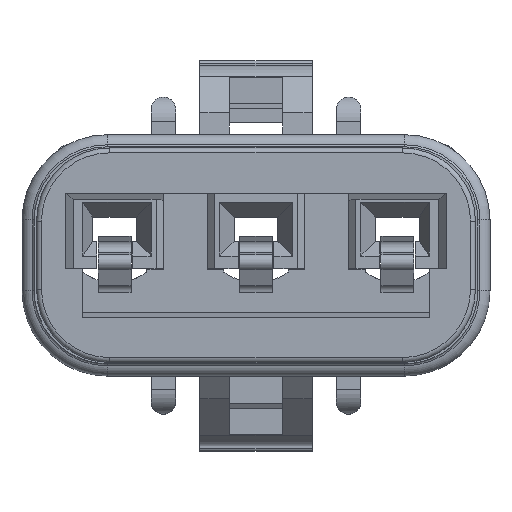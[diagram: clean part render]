
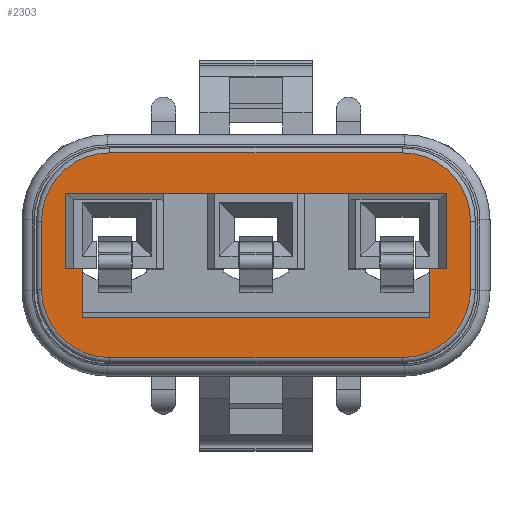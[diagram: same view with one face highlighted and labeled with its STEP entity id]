
A CAD part, top view. The second image highlights one B-rep face of the part: STEP entity #2303.
In plain terms, the highlighted planar face has unit normal (0, 0, 1).
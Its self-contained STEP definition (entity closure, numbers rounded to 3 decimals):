
#38 = LINE ( 'NONE', #7798, #20823 ) ;
#109 = DIRECTION ( 'NONE',  ( 1., 0., 0. ) ) ;
#239 = VERTEX_POINT ( 'NONE', #13555 ) ;
#550 = AXIS2_PLACEMENT_3D ( 'NONE', #7177, #14889, #13173 ) ;
#877 = EDGE_CURVE ( 'NONE', #4485, #15573, #5748, .T. ) ;
#1048 = LINE ( 'NONE', #8560, #22111 ) ;
#1400 = DIRECTION ( 'NONE',  ( 0., 0., 1. ) ) ;
#1514 = VERTEX_POINT ( 'NONE', #10107 ) ;
#1701 = ORIENTED_EDGE ( 'NONE', *, *, #2862, .T. ) ;
#2139 = CIRCLE ( 'NONE', #550, 2.8 ) ;
#2151 = DIRECTION ( 'NONE',  ( 0., 1., 0. ) ) ;
#2303 = ADVANCED_FACE ( 'NONE', ( #15223, #13519 ), #15350, .T. ) ;
#2514 = CARTESIAN_POINT ( 'NONE',  ( 7.125, -0.55, 1.2 ) ) ;
#2654 = DIRECTION ( 'NONE',  ( -1., 0., 0. ) ) ;
#2862 = EDGE_CURVE ( 'NONE', #23455, #21978, #38, .T. ) ;
#3088 = VECTOR ( 'NONE', #14146, 1000. ) ;
#3178 = ORIENTED_EDGE ( 'NONE', *, *, #19509, .T. ) ;
#3377 = CARTESIAN_POINT ( 'NONE',  ( -6., -1.4, 1.2 ) ) ;
#3562 = ORIENTED_EDGE ( 'NONE', *, *, #9195, .T. ) ;
#3669 = EDGE_CURVE ( 'NONE', #9676, #16053, #5112, .T. ) ;
#4128 = DIRECTION ( 'NONE',  ( 1., 0., 0. ) ) ;
#4345 = CARTESIAN_POINT ( 'NONE',  ( -7.825, 2.55, 1.2 ) ) ;
#4485 = VERTEX_POINT ( 'NONE', #19226 ) ;
#4570 = CARTESIAN_POINT ( 'NONE',  ( 3.8, 2.55, 1.2 ) ) ;
#4646 = VERTEX_POINT ( 'NONE', #2514 ) ;
#4940 = DIRECTION ( 'NONE',  ( 1., 0., 0. ) ) ;
#5112 = LINE ( 'NONE', #12576, #19773 ) ;
#5360 = ORIENTED_EDGE ( 'NONE', *, *, #10453, .T. ) ;
#5530 = EDGE_CURVE ( 'NONE', #18386, #4485, #22423, .T. ) ;
#5543 = CIRCLE ( 'NONE', #11796, 2.8 ) ;
#5666 = DIRECTION ( 'NONE',  ( -1., 0., 0. ) ) ;
#5748 = LINE ( 'NONE', #21056, #17946 ) ;
#5795 = DIRECTION ( 'NONE',  ( 0., 0., 1. ) ) ;
#5813 = VECTOR ( 'NONE', #16534, 1000. ) ;
#6271 = EDGE_CURVE ( 'NONE', #23875, #12919, #15872, .T. ) ;
#6560 = DIRECTION ( 'NONE',  ( 0., -1., 0. ) ) ;
#6587 = VERTEX_POINT ( 'NONE', #22367 ) ;
#6703 = VECTOR ( 'NONE', #6560, 1000. ) ;
#7062 = CARTESIAN_POINT ( 'NONE',  ( 6., 1.4, 1.2 ) ) ;
#7071 = CARTESIAN_POINT ( 'NONE',  ( 6., -4.2, 1.2 ) ) ;
#7177 = CARTESIAN_POINT ( 'NONE',  ( 6., -1.4, 1.2 ) ) ;
#7275 = DIRECTION ( 'NONE',  ( 0., -1., 0. ) ) ;
#7515 = VECTOR ( 'NONE', #4128, 1000. ) ;
#7584 = DIRECTION ( 'NONE',  ( 0., 1., 0. ) ) ;
#7798 = CARTESIAN_POINT ( 'NONE',  ( -6., -4.2, 1.2 ) ) ;
#7808 = CARTESIAN_POINT ( 'NONE',  ( 7.125, -2.55, 1.2 ) ) ;
#7863 = VERTEX_POINT ( 'NONE', #8949 ) ;
#8377 = LINE ( 'NONE', #13664, #6703 ) ;
#8509 = CARTESIAN_POINT ( 'NONE',  ( 7.825, 2.55, 1.2 ) ) ;
#8560 = CARTESIAN_POINT ( 'NONE',  ( 7.825, 2.55, 1.2 ) ) ;
#8636 = CARTESIAN_POINT ( 'NONE',  ( -6., -4.2, 1.2 ) ) ;
#8649 = EDGE_CURVE ( 'NONE', #4646, #12919, #12564, .T. ) ;
#8905 = ORIENTED_EDGE ( 'NONE', *, *, #19191, .T. ) ;
#8949 = CARTESIAN_POINT ( 'NONE',  ( 6., 4.2, 1.2 ) ) ;
#8980 = CARTESIAN_POINT ( 'NONE',  ( -7.825, 2.55, 1.2 ) ) ;
#9194 = ORIENTED_EDGE ( 'NONE', *, *, #23990, .T. ) ;
#9195 = EDGE_CURVE ( 'NONE', #7863, #239, #22714, .T. ) ;
#9627 = VERTEX_POINT ( 'NONE', #4570 ) ;
#9676 = VERTEX_POINT ( 'NONE', #8980 ) ;
#9981 = DIRECTION ( 'NONE',  ( 0., -1., 0. ) ) ;
#10107 = CARTESIAN_POINT ( 'NONE',  ( 8.8, 1.4, 1.2 ) ) ;
#10325 = AXIS2_PLACEMENT_3D ( 'NONE', #11915, #5795, #109 ) ;
#10453 = EDGE_CURVE ( 'NONE', #14845, #23455, #21172, .T. ) ;
#10591 = AXIS2_PLACEMENT_3D ( 'NONE', #3377, #1400, #16771 ) ;
#10908 = CARTESIAN_POINT ( 'NONE',  ( -7.825, -0.55, 1.2 ) ) ;
#11796 = AXIS2_PLACEMENT_3D ( 'NONE', #7062, #14649, #14529 ) ;
#11915 = CARTESIAN_POINT ( 'NONE',  ( 0., 0., 1.2 ) ) ;
#12341 = DIRECTION ( 'NONE',  ( 1., 0., 0. ) ) ;
#12399 = ORIENTED_EDGE ( 'NONE', *, *, #8649, .F. ) ;
#12533 = LINE ( 'NONE', #16461, #21524 ) ;
#12564 = LINE ( 'NONE', #23982, #19431 ) ;
#12576 = CARTESIAN_POINT ( 'NONE',  ( -7.825, 2.55, 1.2 ) ) ;
#12788 = CARTESIAN_POINT ( 'NONE',  ( -8.8, 1.4, 1.2 ) ) ;
#12919 = VERTEX_POINT ( 'NONE', #14762 ) ;
#13107 = DIRECTION ( 'NONE',  ( 0., 0., 1. ) ) ;
#13173 = DIRECTION ( 'NONE',  ( 0., -1., 0. ) ) ;
#13327 = DIRECTION ( 'NONE',  ( -1., 0., 0. ) ) ;
#13329 = ORIENTED_EDGE ( 'NONE', *, *, #5530, .T. ) ;
#13334 = ORIENTED_EDGE ( 'NONE', *, *, #877, .T. ) ;
#13519 = FACE_OUTER_BOUND ( 'NONE', #17532, .T. ) ;
#13555 = CARTESIAN_POINT ( 'NONE',  ( -6., 4.2, 1.2 ) ) ;
#13556 = LINE ( 'NONE', #4345, #15757 ) ;
#13664 = CARTESIAN_POINT ( 'NONE',  ( 7.125, -0.55, 1.2 ) ) ;
#13827 = CARTESIAN_POINT ( 'NONE',  ( -7.825, -0.55, 1.2 ) ) ;
#13944 = ORIENTED_EDGE ( 'NONE', *, *, #17935, .T. ) ;
#14146 = DIRECTION ( 'NONE',  ( 0., -1., 0. ) ) ;
#14278 = VECTOR ( 'NONE', #7275, 1000. ) ;
#14529 = DIRECTION ( 'NONE',  ( 1., 0., 0. ) ) ;
#14649 = DIRECTION ( 'NONE',  ( 0., 0., 1. ) ) ;
#14762 = CARTESIAN_POINT ( 'NONE',  ( 7.825, -0.55, 1.2 ) ) ;
#14845 = VERTEX_POINT ( 'NONE', #19666 ) ;
#14889 = DIRECTION ( 'NONE',  ( 0., 0., 1. ) ) ;
#14981 = ORIENTED_EDGE ( 'NONE', *, *, #16760, .T. ) ;
#15223 = FACE_BOUND ( 'NONE', #17785, .T. ) ;
#15350 = PLANE ( 'NONE',  #10325 ) ;
#15539 = ORIENTED_EDGE ( 'NONE', *, *, #20038, .F. ) ;
#15573 = VERTEX_POINT ( 'NONE', #17230 ) ;
#15757 = VECTOR ( 'NONE', #9981, 1000. ) ;
#15872 = LINE ( 'NONE', #8509, #3088 ) ;
#16053 = VERTEX_POINT ( 'NONE', #18349 ) ;
#16461 = CARTESIAN_POINT ( 'NONE',  ( -3.8, 2.55, 1.2 ) ) ;
#16534 = DIRECTION ( 'NONE',  ( 0., 1., 0. ) ) ;
#16760 = EDGE_CURVE ( 'NONE', #22940, #1514, #18366, .T. ) ;
#16771 = DIRECTION ( 'NONE',  ( -1., 0., 0. ) ) ;
#17230 = CARTESIAN_POINT ( 'NONE',  ( -7.125, -0.55, 1.2 ) ) ;
#17297 = CIRCLE ( 'NONE', #19259, 2.8 ) ;
#17355 = VERTEX_POINT ( 'NONE', #10908 ) ;
#17377 = LINE ( 'NONE', #13827, #7515 ) ;
#17532 = EDGE_LOOP ( 'NONE', ( #8905, #3562, #3178, #9194, #5360, #1701, #21529, #14981 ) ) ;
#17785 = EDGE_LOOP ( 'NONE', ( #13334, #18078, #15539, #18946, #13944, #22602, #24134, #12399, #18398, #13329 ) ) ;
#17935 = EDGE_CURVE ( 'NONE', #16053, #9627, #12533, .T. ) ;
#17946 = VECTOR ( 'NONE', #7584, 1000. ) ;
#18078 = ORIENTED_EDGE ( 'NONE', *, *, #19645, .F. ) ;
#18349 = CARTESIAN_POINT ( 'NONE',  ( -3.8, 2.55, 1.2 ) ) ;
#18366 = LINE ( 'NONE', #20446, #5813 ) ;
#18386 = VERTEX_POINT ( 'NONE', #19620 ) ;
#18398 = ORIENTED_EDGE ( 'NONE', *, *, #18498, .T. ) ;
#18451 = DIRECTION ( 'NONE',  ( 1., 0., 0. ) ) ;
#18498 = EDGE_CURVE ( 'NONE', #4646, #18386, #8377, .T. ) ;
#18946 = ORIENTED_EDGE ( 'NONE', *, *, #3669, .T. ) ;
#18981 = CARTESIAN_POINT ( 'NONE',  ( -6., 1.4, 1.2 ) ) ;
#19030 = CARTESIAN_POINT ( 'NONE',  ( 6., 4.2, 1.2 ) ) ;
#19146 = VECTOR ( 'NONE', #13327, 1000. ) ;
#19191 = EDGE_CURVE ( 'NONE', #1514, #7863, #5543, .T. ) ;
#19226 = CARTESIAN_POINT ( 'NONE',  ( -7.125, -2.55, 1.2 ) ) ;
#19259 = AXIS2_PLACEMENT_3D ( 'NONE', #18981, #13107, #2151 ) ;
#19431 = VECTOR ( 'NONE', #18451, 1000. ) ;
#19509 = EDGE_CURVE ( 'NONE', #239, #6587, #17297, .T. ) ;
#19512 = CARTESIAN_POINT ( 'NONE',  ( 8.8, -1.4, 1.2 ) ) ;
#19620 = CARTESIAN_POINT ( 'NONE',  ( 7.125, -2.55, 1.2 ) ) ;
#19645 = EDGE_CURVE ( 'NONE', #17355, #15573, #17377, .T. ) ;
#19666 = CARTESIAN_POINT ( 'NONE',  ( -8.8, -1.4, 1.2 ) ) ;
#19773 = VECTOR ( 'NONE', #12341, 1000. ) ;
#20038 = EDGE_CURVE ( 'NONE', #9676, #17355, #13556, .T. ) ;
#20446 = CARTESIAN_POINT ( 'NONE',  ( 8.8, -1.4, 1.2 ) ) ;
#20673 = DIRECTION ( 'NONE',  ( 1., 0., 0. ) ) ;
#20823 = VECTOR ( 'NONE', #20673, 1000. ) ;
#21056 = CARTESIAN_POINT ( 'NONE',  ( -7.125, -2.55, 1.2 ) ) ;
#21172 = CIRCLE ( 'NONE', #10591, 2.8 ) ;
#21524 = VECTOR ( 'NONE', #4940, 1000. ) ;
#21529 = ORIENTED_EDGE ( 'NONE', *, *, #24176, .T. ) ;
#21978 = VERTEX_POINT ( 'NONE', #7071 ) ;
#22103 = LINE ( 'NONE', #12788, #14278 ) ;
#22111 = VECTOR ( 'NONE', #2654, 1000. ) ;
#22193 = VECTOR ( 'NONE', #5666, 1000. ) ;
#22367 = CARTESIAN_POINT ( 'NONE',  ( -8.8, 1.4, 1.2 ) ) ;
#22423 = LINE ( 'NONE', #7808, #19146 ) ;
#22602 = ORIENTED_EDGE ( 'NONE', *, *, #23257, .F. ) ;
#22714 = LINE ( 'NONE', #19030, #22193 ) ;
#22940 = VERTEX_POINT ( 'NONE', #19512 ) ;
#23111 = CARTESIAN_POINT ( 'NONE',  ( 7.825, 2.55, 1.2 ) ) ;
#23257 = EDGE_CURVE ( 'NONE', #23875, #9627, #1048, .T. ) ;
#23455 = VERTEX_POINT ( 'NONE', #8636 ) ;
#23875 = VERTEX_POINT ( 'NONE', #23111 ) ;
#23982 = CARTESIAN_POINT ( 'NONE',  ( 7.125, -0.55, 1.2 ) ) ;
#23990 = EDGE_CURVE ( 'NONE', #6587, #14845, #22103, .T. ) ;
#24134 = ORIENTED_EDGE ( 'NONE', *, *, #6271, .T. ) ;
#24176 = EDGE_CURVE ( 'NONE', #21978, #22940, #2139, .T. ) ;
